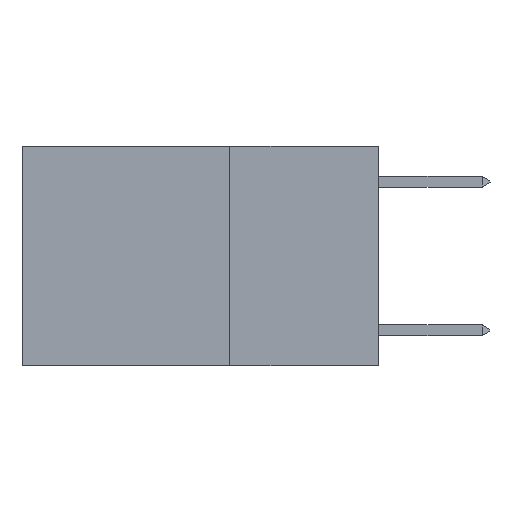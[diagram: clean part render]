
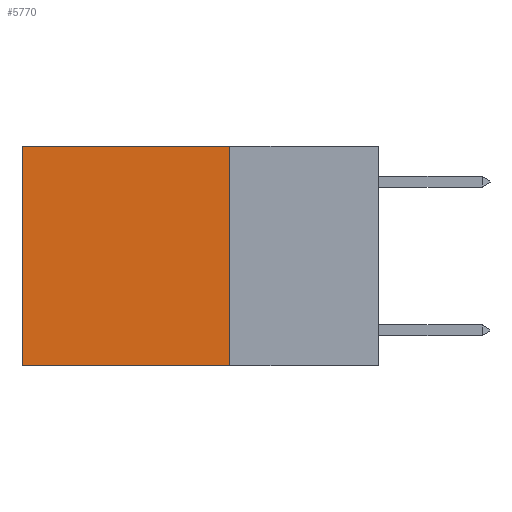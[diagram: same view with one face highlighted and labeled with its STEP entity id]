
A CAD part, left-side view. The second image highlights one B-rep face of the part: STEP entity #5770.
In plain terms, the highlighted planar face has unit normal (-1, 0, 0).
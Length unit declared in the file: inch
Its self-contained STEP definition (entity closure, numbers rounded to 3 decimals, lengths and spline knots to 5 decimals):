
#96 = LINE ( 'NONE', #1179, #1841 ) ;
#190 = VERTEX_POINT ( 'NONE', #2668 ) ;
#1076 = CARTESIAN_POINT ( 'NONE',  ( 0.2625, 0.25, -0.37 ) ) ;
#1136 = PLANE ( 'NONE',  #8101 ) ;
#1162 = CARTESIAN_POINT ( 'NONE',  ( 0.2625, 0.6, -0.37 ) ) ;
#1179 = CARTESIAN_POINT ( 'NONE',  ( 0.2625, 0.25, 0. ) ) ;
#1495 = VERTEX_POINT ( 'NONE', #3748 ) ;
#1758 = DIRECTION ( 'NONE',  ( 0., 1., 0. ) ) ;
#1841 = VECTOR ( 'NONE', #6066, 39.37008 ) ;
#2119 = EDGE_CURVE ( 'NONE', #1495, #5787, #5628, .T. ) ;
#2391 = DIRECTION ( 'NONE',  ( 0., 0., -1. ) ) ;
#2577 = CARTESIAN_POINT ( 'NONE',  ( 0.2625, 0.25, 0. ) ) ;
#2668 = CARTESIAN_POINT ( 'NONE',  ( 0.2625, 0.25, 0. ) ) ;
#2973 = VECTOR ( 'NONE', #2391, 39.37008 ) ;
#3302 = EDGE_CURVE ( 'NONE', #7183, #5787, #8753, .T. ) ;
#3307 = DIRECTION ( 'NONE',  ( 0., 0., -1. ) ) ;
#3427 = CARTESIAN_POINT ( 'NONE',  ( 0.2625, 0.6, 0. ) ) ;
#3592 = VECTOR ( 'NONE', #4181, 39.37008 ) ;
#3748 = CARTESIAN_POINT ( 'NONE',  ( 0.2625, 0.6, 0. ) ) ;
#3884 = EDGE_LOOP ( 'NONE', ( #8644, #8677, #8700, #8715 ) ) ;
#4181 = DIRECTION ( 'NONE',  ( 0., 0., -1. ) ) ;
#5066 = EDGE_CURVE ( 'NONE', #190, #1495, #96, .T. ) ;
#5360 = FACE_OUTER_BOUND ( 'NONE', #3884, .T. ) ;
#5555 = EDGE_CURVE ( 'NONE', #190, #7183, #6626, .T. ) ;
#5628 = LINE ( 'NONE', #3427, #3592 ) ;
#5770 = ADVANCED_FACE ( 'NONE', ( #5360 ), #1136, .F. ) ;
#5787 = VERTEX_POINT ( 'NONE', #1162 ) ;
#6066 = DIRECTION ( 'NONE',  ( 0., 1., 0. ) ) ;
#6454 = CARTESIAN_POINT ( 'NONE',  ( 0.2625, 0.25, -0.37 ) ) ;
#6542 = CARTESIAN_POINT ( 'NONE',  ( 0.2625, 0.25, 0. ) ) ;
#6626 = LINE ( 'NONE', #6542, #2973 ) ;
#7183 = VERTEX_POINT ( 'NONE', #6454 ) ;
#7381 = DIRECTION ( 'NONE',  ( 1., 0., 0. ) ) ;
#8101 = AXIS2_PLACEMENT_3D ( 'NONE', #2577, #7381, #3307 ) ;
#8381 = VECTOR ( 'NONE', #1758, 39.37008 ) ;
#8644 = ORIENTED_EDGE ( 'NONE', *, *, #2119, .T. ) ;
#8677 = ORIENTED_EDGE ( 'NONE', *, *, #3302, .F. ) ;
#8700 = ORIENTED_EDGE ( 'NONE', *, *, #5555, .F. ) ;
#8715 = ORIENTED_EDGE ( 'NONE', *, *, #5066, .T. ) ;
#8753 = LINE ( 'NONE', #1076, #8381 ) ;
